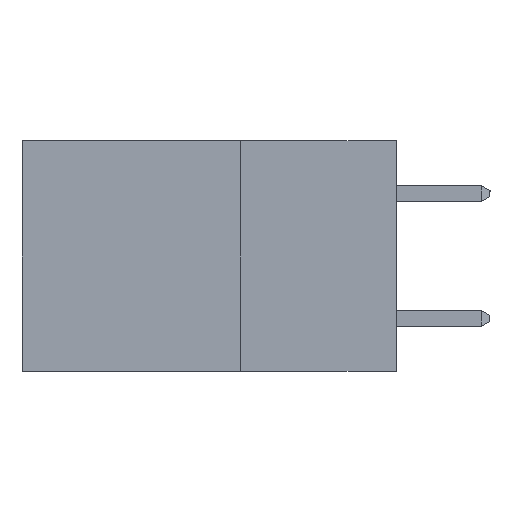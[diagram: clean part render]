
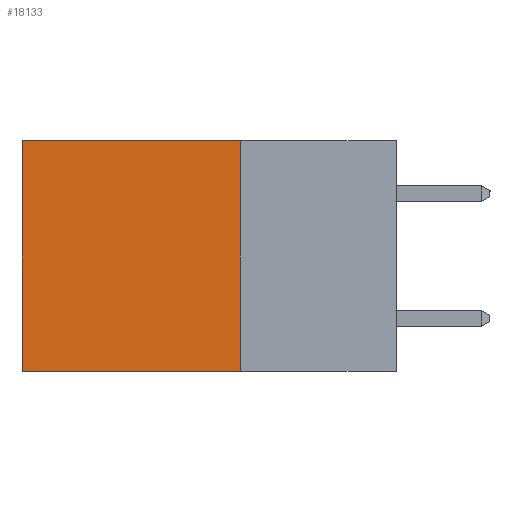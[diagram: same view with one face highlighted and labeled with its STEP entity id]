
A CAD part, left-side view. The second image highlights one B-rep face of the part: STEP entity #18133.
In plain terms, the highlighted planar face has unit normal (-1, 0, 0).
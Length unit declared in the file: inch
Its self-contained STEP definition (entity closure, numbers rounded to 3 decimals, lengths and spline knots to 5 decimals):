
#835 = PLANE ( 'NONE',  #5827 ) ;
#1019 = CARTESIAN_POINT ( 'NONE',  ( 0.2615, 0.6, 0. ) ) ;
#1590 = DIRECTION ( 'NONE',  ( 0., 1., 0. ) ) ;
#1630 = LINE ( 'NONE', #6517, #16073 ) ;
#1730 = CARTESIAN_POINT ( 'NONE',  ( 0.2615, 0.6, -0.37 ) ) ;
#2291 = EDGE_LOOP ( 'NONE', ( #20593, #21163, #13804, #20608 ) ) ;
#3023 = DIRECTION ( 'NONE',  ( 0., 1., 0. ) ) ;
#3364 = EDGE_CURVE ( 'NONE', #17946, #16141, #12055, .T. ) ;
#3525 = LINE ( 'NONE', #17618, #7978 ) ;
#4722 = VECTOR ( 'NONE', #21379, 39.37008 ) ;
#5827 = AXIS2_PLACEMENT_3D ( 'NONE', #11060, #14589, #16293 ) ;
#5994 = CARTESIAN_POINT ( 'NONE',  ( 0.2615, 0.6, -0.37 ) ) ;
#6517 = CARTESIAN_POINT ( 'NONE',  ( 0.2615, 0.25, 0. ) ) ;
#6583 = EDGE_CURVE ( 'NONE', #9148, #16821, #7680, .T. ) ;
#7680 = LINE ( 'NONE', #5994, #9012 ) ;
#7978 = VECTOR ( 'NONE', #1590, 39.37008 ) ;
#8050 = CARTESIAN_POINT ( 'NONE',  ( 0.2615, 0.25, -0.37 ) ) ;
#8316 = EDGE_CURVE ( 'NONE', #16141, #16821, #3525, .T. ) ;
#9012 = VECTOR ( 'NONE', #12915, 39.37008 ) ;
#9148 = VERTEX_POINT ( 'NONE', #1019 ) ;
#10140 = CARTESIAN_POINT ( 'NONE',  ( 0.2615, 0.25, 0. ) ) ;
#11060 = CARTESIAN_POINT ( 'NONE',  ( 0.2615, 0.25, -0.37 ) ) ;
#12055 = LINE ( 'NONE', #19694, #4722 ) ;
#12529 = FACE_OUTER_BOUND ( 'NONE', #2291, .T. ) ;
#12915 = DIRECTION ( 'NONE',  ( 0., 0., -1. ) ) ;
#13804 = ORIENTED_EDGE ( 'NONE', *, *, #3364, .F. ) ;
#14589 = DIRECTION ( 'NONE',  ( 1., 0., 0. ) ) ;
#16073 = VECTOR ( 'NONE', #3023, 39.37008 ) ;
#16141 = VERTEX_POINT ( 'NONE', #8050 ) ;
#16293 = DIRECTION ( 'NONE',  ( 0., 0., -1. ) ) ;
#16821 = VERTEX_POINT ( 'NONE', #1730 ) ;
#17618 = CARTESIAN_POINT ( 'NONE',  ( 0.2615, 0.25, -0.37 ) ) ;
#17946 = VERTEX_POINT ( 'NONE', #10140 ) ;
#18133 = ADVANCED_FACE ( 'NONE', ( #12529 ), #835, .F. ) ;
#19694 = CARTESIAN_POINT ( 'NONE',  ( 0.2615, 0.25, -0.37 ) ) ;
#20110 = EDGE_CURVE ( 'NONE', #17946, #9148, #1630, .T. ) ;
#20593 = ORIENTED_EDGE ( 'NONE', *, *, #6583, .T. ) ;
#20608 = ORIENTED_EDGE ( 'NONE', *, *, #20110, .T. ) ;
#21163 = ORIENTED_EDGE ( 'NONE', *, *, #8316, .F. ) ;
#21379 = DIRECTION ( 'NONE',  ( 0., 0., -1. ) ) ;
